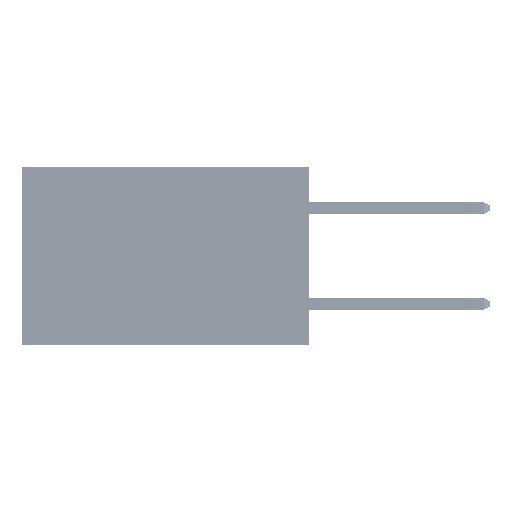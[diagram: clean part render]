
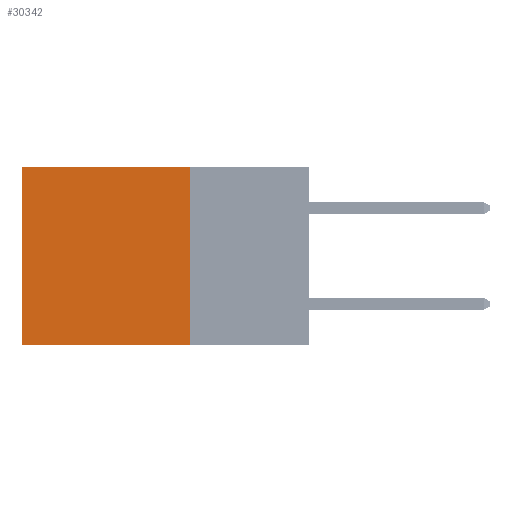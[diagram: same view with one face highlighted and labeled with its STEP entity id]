
A CAD part, left-side view. The second image highlights one B-rep face of the part: STEP entity #30342.
In plain terms, the highlighted planar face has unit normal (-1, 0, 0).
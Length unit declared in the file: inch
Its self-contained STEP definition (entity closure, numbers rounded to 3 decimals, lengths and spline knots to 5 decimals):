
#1193 = EDGE_CURVE ( 'NONE', #50134, #49916, #21240, .T. ) ;
#2688 = EDGE_LOOP ( 'NONE', ( #45722, #51266, #26810, #41782 ) ) ;
#9776 = VECTOR ( 'NONE', #46970, 39.37008 ) ;
#11761 = VECTOR ( 'NONE', #19580, 39.37008 ) ;
#12196 = CARTESIAN_POINT ( 'NONE',  ( 0.2875, 0.25, 0. ) ) ;
#16291 = LINE ( 'NONE', #22588, #36427 ) ;
#17769 = CARTESIAN_POINT ( 'NONE',  ( 0.2875, 0.25, 0. ) ) ;
#18706 = CARTESIAN_POINT ( 'NONE',  ( 0.2875, 0.25, -0.37 ) ) ;
#19580 = DIRECTION ( 'NONE',  ( 0., 0., -1. ) ) ;
#20420 = DIRECTION ( 'NONE',  ( 1., 0., 0. ) ) ;
#21240 = LINE ( 'NONE', #18706, #50625 ) ;
#21341 = LINE ( 'NONE', #35536, #11761 ) ;
#21426 = VERTEX_POINT ( 'NONE', #17769 ) ;
#21855 = FACE_OUTER_BOUND ( 'NONE', #2688, .T. ) ;
#22172 = EDGE_CURVE ( 'NONE', #41302, #49916, #31361, .T. ) ;
#22588 = CARTESIAN_POINT ( 'NONE',  ( 0.2875, 0.25, 0. ) ) ;
#22938 = DIRECTION ( 'NONE',  ( 0., 1., 0. ) ) ;
#26618 = DIRECTION ( 'NONE',  ( 0., 1., 0. ) ) ;
#26810 = ORIENTED_EDGE ( 'NONE', *, *, #45843, .F. ) ;
#27685 = CARTESIAN_POINT ( 'NONE',  ( 0.2875, 0.6, 0. ) ) ;
#30342 = ADVANCED_FACE ( 'NONE', ( #21855 ), #52262, .F. ) ;
#31361 = LINE ( 'NONE', #38924, #9776 ) ;
#32882 = CARTESIAN_POINT ( 'NONE',  ( 0.2875, 0.25, -0.37 ) ) ;
#34422 = EDGE_CURVE ( 'NONE', #21426, #41302, #16291, .T. ) ;
#35536 = CARTESIAN_POINT ( 'NONE',  ( 0.2875, 0.25, 0. ) ) ;
#36080 = AXIS2_PLACEMENT_3D ( 'NONE', #12196, #20420, #48388 ) ;
#36427 = VECTOR ( 'NONE', #26618, 39.37008 ) ;
#38924 = CARTESIAN_POINT ( 'NONE',  ( 0.2875, 0.6, 0. ) ) ;
#41302 = VERTEX_POINT ( 'NONE', #27685 ) ;
#41782 = ORIENTED_EDGE ( 'NONE', *, *, #34422, .T. ) ;
#43522 = CARTESIAN_POINT ( 'NONE',  ( 0.2875, 0.6, -0.37 ) ) ;
#45722 = ORIENTED_EDGE ( 'NONE', *, *, #22172, .T. ) ;
#45843 = EDGE_CURVE ( 'NONE', #21426, #50134, #21341, .T. ) ;
#46970 = DIRECTION ( 'NONE',  ( 0., 0., -1. ) ) ;
#48388 = DIRECTION ( 'NONE',  ( 0., 0., -1. ) ) ;
#49916 = VERTEX_POINT ( 'NONE', #43522 ) ;
#50134 = VERTEX_POINT ( 'NONE', #32882 ) ;
#50625 = VECTOR ( 'NONE', #22938, 39.37008 ) ;
#51266 = ORIENTED_EDGE ( 'NONE', *, *, #1193, .F. ) ;
#52262 = PLANE ( 'NONE',  #36080 ) ;
